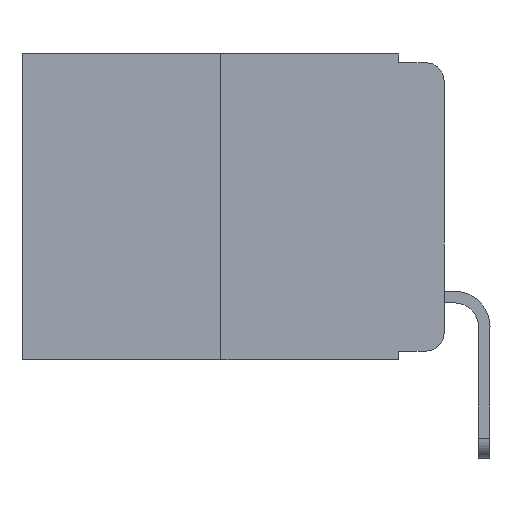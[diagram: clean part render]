
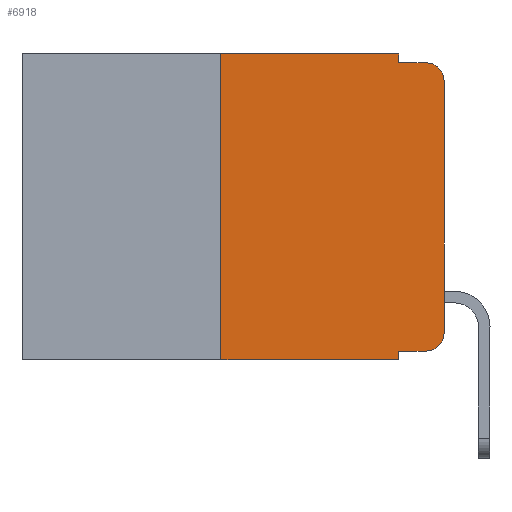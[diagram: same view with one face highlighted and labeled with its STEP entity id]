
A CAD part, left-side view. The second image highlights one B-rep face of the part: STEP entity #6918.
In plain terms, the highlighted planar face has unit normal (-1, 0, 0).
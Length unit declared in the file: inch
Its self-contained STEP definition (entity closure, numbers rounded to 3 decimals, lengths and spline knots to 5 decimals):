
#5 = VERTEX_POINT ( 'NONE', #19294 ) ;
#84 = CARTESIAN_POINT ( 'NONE',  ( 0., 0.02, -0.01 ) ) ;
#240 = LINE ( 'NONE', #9873, #4262 ) ;
#265 = VERTEX_POINT ( 'NONE', #18702 ) ;
#740 = ORIENTED_EDGE ( 'NONE', *, *, #12745, .F. ) ;
#1049 = LINE ( 'NONE', #10192, #13633 ) ;
#2296 = LINE ( 'NONE', #8169, #13317 ) ;
#2568 = VECTOR ( 'NONE', #5299, 39.37008 ) ;
#2627 = CARTESIAN_POINT ( 'NONE',  ( 0., 0.051, 0. ) ) ;
#2639 = CARTESIAN_POINT ( 'NONE',  ( 0., 0.051, -0.333 ) ) ;
#2982 = CARTESIAN_POINT ( 'NONE',  ( 0., 0., -0.313 ) ) ;
#3137 = EDGE_CURVE ( 'NONE', #10313, #17986, #6289, .T. ) ;
#3150 = ORIENTED_EDGE ( 'NONE', *, *, #16750, .T. ) ;
#3173 = DIRECTION ( 'NONE',  ( 0., 0., 1. ) ) ;
#3250 = DIRECTION ( 'NONE',  ( 0., 0., -1. ) ) ;
#3430 = EDGE_CURVE ( 'NONE', #17348, #6515, #3893, .T. ) ;
#3593 = ORIENTED_EDGE ( 'NONE', *, *, #3137, .T. ) ;
#3662 = CARTESIAN_POINT ( 'NONE',  ( 0., 0., 0. ) ) ;
#3893 = LINE ( 'NONE', #16099, #16122 ) ;
#4262 = VECTOR ( 'NONE', #3250, 39.37008 ) ;
#4419 = ORIENTED_EDGE ( 'NONE', *, *, #11712, .F. ) ;
#4657 = VERTEX_POINT ( 'NONE', #11657 ) ;
#4738 = CARTESIAN_POINT ( 'NONE',  ( 0., 0.02, -0.03 ) ) ;
#5010 = CARTESIAN_POINT ( 'NONE',  ( 0., 0.02, -0.313 ) ) ;
#5116 = VERTEX_POINT ( 'NONE', #2982 ) ;
#5299 = DIRECTION ( 'NONE',  ( 0., 0., 1. ) ) ;
#5835 = VECTOR ( 'NONE', #20091, 39.37008 ) ;
#6245 = CARTESIAN_POINT ( 'NONE',  ( 0., 0.473, -0.343 ) ) ;
#6289 = LINE ( 'NONE', #6245, #9625 ) ;
#6433 = DIRECTION ( 'NONE',  ( 0., 0., -1. ) ) ;
#6515 = VERTEX_POINT ( 'NONE', #2627 ) ;
#6580 = LINE ( 'NONE', #16650, #19023 ) ;
#6704 = DIRECTION ( 'NONE',  ( 0., 0., -1. ) ) ;
#6918 = ADVANCED_FACE ( 'NONE', ( #19304 ), #17555, .F. ) ;
#7804 = CIRCLE ( 'NONE', #11069, 0.02 ) ;
#8011 = VERTEX_POINT ( 'NONE', #84 ) ;
#8169 = CARTESIAN_POINT ( 'NONE',  ( 0., 0.25, 0. ) ) ;
#8570 = CARTESIAN_POINT ( 'NONE',  ( 0., 0.051, -0.343 ) ) ;
#8945 = DIRECTION ( 'NONE',  ( 0., 0., -1. ) ) ;
#9553 = EDGE_CURVE ( 'NONE', #265, #5116, #7804, .T. ) ;
#9606 = DIRECTION ( 'NONE',  ( 0., -1., 0. ) ) ;
#9625 = VECTOR ( 'NONE', #9606, 39.37008 ) ;
#9873 = CARTESIAN_POINT ( 'NONE',  ( 0., 0.051, 0. ) ) ;
#10172 = ORIENTED_EDGE ( 'NONE', *, *, #14796, .F. ) ;
#10192 = CARTESIAN_POINT ( 'NONE',  ( 0., 0.051, -0.01 ) ) ;
#10313 = VERTEX_POINT ( 'NONE', #15407 ) ;
#10412 = CIRCLE ( 'NONE', #10625, 0.02 ) ;
#10625 = AXIS2_PLACEMENT_3D ( 'NONE', #4738, #15860, #6433 ) ;
#10633 = EDGE_CURVE ( 'NONE', #20445, #265, #15279, .T. ) ;
#11069 = AXIS2_PLACEMENT_3D ( 'NONE', #5010, #16102, #6704 ) ;
#11477 = CARTESIAN_POINT ( 'NONE',  ( 0., 0.473, 0. ) ) ;
#11539 = DIRECTION ( 'NONE',  ( 0., 0., -1. ) ) ;
#11657 = CARTESIAN_POINT ( 'NONE',  ( 0., 0.051, -0.01 ) ) ;
#11712 = EDGE_CURVE ( 'NONE', #20445, #17986, #6580, .T. ) ;
#11818 = DIRECTION ( 'NONE',  ( 0., -1., 0. ) ) ;
#11888 = LINE ( 'NONE', #3662, #2568 ) ;
#12745 = EDGE_CURVE ( 'NONE', #10313, #17348, #2296, .T. ) ;
#13317 = VECTOR ( 'NONE', #3173, 39.37008 ) ;
#13633 = VECTOR ( 'NONE', #11818, 39.37008 ) ;
#13766 = EDGE_CURVE ( 'NONE', #6515, #4657, #240, .T. ) ;
#14474 = EDGE_LOOP ( 'NONE', ( #3150, #15943, #10172, #18319, #15261, #740, #3593, #4419, #15538, #15703 ) ) ;
#14796 = EDGE_CURVE ( 'NONE', #4657, #8011, #1049, .T. ) ;
#15261 = ORIENTED_EDGE ( 'NONE', *, *, #3430, .F. ) ;
#15279 = LINE ( 'NONE', #2639, #5835 ) ;
#15407 = CARTESIAN_POINT ( 'NONE',  ( 0., 0.25, -0.343 ) ) ;
#15538 = ORIENTED_EDGE ( 'NONE', *, *, #10633, .T. ) ;
#15703 = ORIENTED_EDGE ( 'NONE', *, *, #9553, .T. ) ;
#15765 = EDGE_CURVE ( 'NONE', #5, #8011, #10412, .T. ) ;
#15860 = DIRECTION ( 'NONE',  ( -1., 0., 0. ) ) ;
#15943 = ORIENTED_EDGE ( 'NONE', *, *, #15765, .T. ) ;
#16099 = CARTESIAN_POINT ( 'NONE',  ( 0., 0.473, 0. ) ) ;
#16101 = DIRECTION ( 'NONE',  ( 0., -1., 0. ) ) ;
#16102 = DIRECTION ( 'NONE',  ( -1., 0., 0. ) ) ;
#16122 = VECTOR ( 'NONE', #16101, 39.37008 ) ;
#16650 = CARTESIAN_POINT ( 'NONE',  ( 0., 0.051, 0. ) ) ;
#16750 = EDGE_CURVE ( 'NONE', #5116, #5, #11888, .T. ) ;
#17300 = CARTESIAN_POINT ( 'NONE',  ( 0., 0.051, -0.333 ) ) ;
#17348 = VERTEX_POINT ( 'NONE', #18185 ) ;
#17555 = PLANE ( 'NONE',  #19445 ) ;
#17986 = VERTEX_POINT ( 'NONE', #8570 ) ;
#18185 = CARTESIAN_POINT ( 'NONE',  ( 0., 0.25, 0. ) ) ;
#18319 = ORIENTED_EDGE ( 'NONE', *, *, #13766, .F. ) ;
#18702 = CARTESIAN_POINT ( 'NONE',  ( 0., 0.02, -0.333 ) ) ;
#19023 = VECTOR ( 'NONE', #8945, 39.37008 ) ;
#19294 = CARTESIAN_POINT ( 'NONE',  ( 0., 0., -0.03 ) ) ;
#19304 = FACE_OUTER_BOUND ( 'NONE', #14474, .T. ) ;
#19445 = AXIS2_PLACEMENT_3D ( 'NONE', #11477, #20614, #11539 ) ;
#20091 = DIRECTION ( 'NONE',  ( 0., -1., 0. ) ) ;
#20445 = VERTEX_POINT ( 'NONE', #17300 ) ;
#20614 = DIRECTION ( 'NONE',  ( 1., 0., 0. ) ) ;
